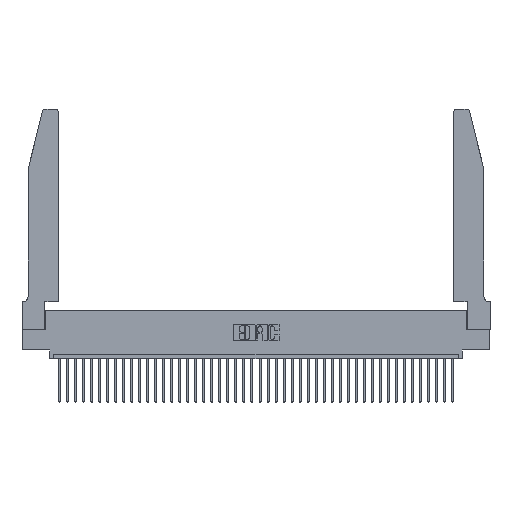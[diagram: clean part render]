
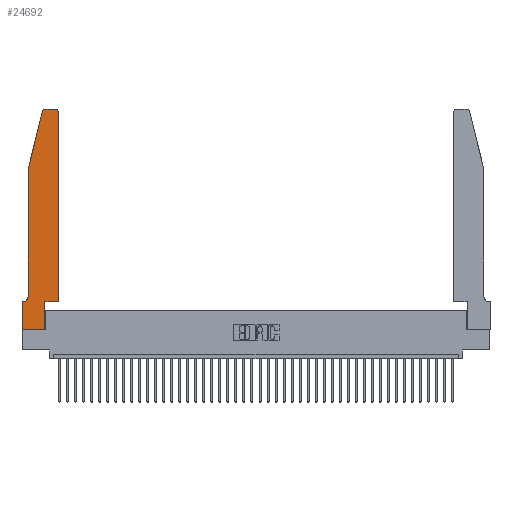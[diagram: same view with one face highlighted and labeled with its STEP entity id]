
A CAD part, top view. The second image highlights one B-rep face of the part: STEP entity #24692.
In plain terms, the highlighted planar face has unit normal (0, 0, 1).
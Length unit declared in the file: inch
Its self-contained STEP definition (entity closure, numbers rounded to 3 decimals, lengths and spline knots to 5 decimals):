
#1592 = VERTEX_POINT ( 'NONE', #25373 ) ;
#1795 = DIRECTION ( 'NONE',  ( 1., 0., 0. ) ) ;
#1961 = VERTEX_POINT ( 'NONE', #6447 ) ;
#2151 = CARTESIAN_POINT ( 'NONE',  ( 0.4205, 2.72, 0.37 ) ) ;
#2471 = CARTESIAN_POINT ( 'NONE',  ( 0.0755, 0.42, 0.37 ) ) ;
#2790 = LINE ( 'NONE', #35418, #9738 ) ;
#3398 = LINE ( 'NONE', #11113, #10912 ) ;
#3417 = ORIENTED_EDGE ( 'NONE', *, *, #31023, .T. ) ;
#3497 = VECTOR ( 'NONE', #39187, 39.37008 ) ;
#4073 = AXIS2_PLACEMENT_3D ( 'NONE', #36904, #4329, #7542 ) ;
#4329 = DIRECTION ( 'NONE',  ( 0., 0., 1. ) ) ;
#6447 = CARTESIAN_POINT ( 'NONE',  ( 0.0055, 0.35, 0.37 ) ) ;
#7184 = EDGE_CURVE ( 'NONE', #39965, #19080, #30500, .T. ) ;
#7542 = DIRECTION ( 'NONE',  ( 1., 0., 0. ) ) ;
#8262 = DIRECTION ( 'NONE',  ( 0., 0., 1. ) ) ;
#8301 = LINE ( 'NONE', #34296, #31265 ) ;
#8438 = DIRECTION ( 'NONE',  ( 1., 0., 0. ) ) ;
#8507 = DIRECTION ( 'NONE',  ( 0., -1., 0. ) ) ;
#8830 = CIRCLE ( 'NONE', #4073, 0.03 ) ;
#9182 = ORIENTED_EDGE ( 'NONE', *, *, #26389, .T. ) ;
#9738 = VECTOR ( 'NONE', #22558, 39.37008 ) ;
#9892 = CARTESIAN_POINT ( 'NONE',  ( 0.0755, 2., 0.37 ) ) ;
#10558 = VERTEX_POINT ( 'NONE', #12761 ) ;
#10912 = VECTOR ( 'NONE', #26677, 39.37008 ) ;
#10990 = LINE ( 'NONE', #30282, #27464 ) ;
#11113 = CARTESIAN_POINT ( 'NONE',  ( 0.4505, 0.35, 0.37 ) ) ;
#11915 = CARTESIAN_POINT ( 'NONE',  ( 0.284, 2.75, 0.37 ) ) ;
#12387 = ORIENTED_EDGE ( 'NONE', *, *, #39981, .T. ) ;
#12761 = CARTESIAN_POINT ( 'NONE',  ( 0.4505, 2.72, 0.37 ) ) ;
#13233 = CARTESIAN_POINT ( 'NONE',  ( 0., 0., 0.37 ) ) ;
#13507 = VECTOR ( 'NONE', #8507, 39.37008 ) ;
#13858 = AXIS2_PLACEMENT_3D ( 'NONE', #2151, #27553, #8438 ) ;
#14632 = AXIS2_PLACEMENT_3D ( 'NONE', #34479, #18452, #25092 ) ;
#15091 = CARTESIAN_POINT ( 'NONE',  ( 0., 0.35, 0.37 ) ) ;
#15648 = ORIENTED_EDGE ( 'NONE', *, *, #28851, .T. ) ;
#16518 = CARTESIAN_POINT ( 'NONE',  ( 0.25487, 2.72718, 0.37 ) ) ;
#17806 = EDGE_CURVE ( 'NONE', #23281, #10558, #3398, .T. ) ;
#17874 = LINE ( 'NONE', #36622, #32758 ) ;
#18004 = CARTESIAN_POINT ( 'NONE',  ( 0., 0., 0.37 ) ) ;
#18163 = CARTESIAN_POINT ( 'NONE',  ( 0.4505, 0.35, 0.37 ) ) ;
#18452 = DIRECTION ( 'NONE',  ( 0., 0., -1. ) ) ;
#18645 = ORIENTED_EDGE ( 'NONE', *, *, #27045, .T. ) ;
#18947 = CIRCLE ( 'NONE', #14632, 0.07 ) ;
#19080 = VERTEX_POINT ( 'NONE', #2471 ) ;
#19189 = EDGE_CURVE ( 'NONE', #30478, #39965, #17874, .T. ) ;
#19317 = CARTESIAN_POINT ( 'NONE',  ( 0.2865, 0.35, 0.37 ) ) ;
#19627 = LINE ( 'NONE', #39308, #32118 ) ;
#19789 = AXIS2_PLACEMENT_3D ( 'NONE', #15091, #8262, #1795 ) ;
#20013 = LINE ( 'NONE', #13233, #3497 ) ;
#20173 = CIRCLE ( 'NONE', #13858, 0.03 ) ;
#20336 = ORIENTED_EDGE ( 'NONE', *, *, #17806, .T. ) ;
#20434 = VERTEX_POINT ( 'NONE', #40212 ) ;
#20573 = VERTEX_POINT ( 'NONE', #18004 ) ;
#20961 = DIRECTION ( 'NONE',  ( 1., 0., 0. ) ) ;
#21600 = EDGE_CURVE ( 'NONE', #1592, #28769, #19627, .T. ) ;
#22558 = DIRECTION ( 'NONE',  ( -1., 0., 0. ) ) ;
#23281 = VERTEX_POINT ( 'NONE', #18163 ) ;
#23742 = DIRECTION ( 'NONE',  ( -0.239, -0.971, 0. ) ) ;
#24692 = ADVANCED_FACE ( 'NONE', ( #34099 ), #40645, .T. ) ;
#25053 = DIRECTION ( 'NONE',  ( 1., 0., 0. ) ) ;
#25092 = DIRECTION ( 'NONE',  ( -1., 0., 0. ) ) ;
#25373 = CARTESIAN_POINT ( 'NONE',  ( 0.2865, 0., 0.37 ) ) ;
#25801 = VERTEX_POINT ( 'NONE', #26872 ) ;
#26389 = EDGE_CURVE ( 'NONE', #20434, #20573, #20013, .T. ) ;
#26576 = DIRECTION ( 'NONE',  ( 0., 1., 0. ) ) ;
#26677 = DIRECTION ( 'NONE',  ( 0., 1., 0. ) ) ;
#26872 = CARTESIAN_POINT ( 'NONE',  ( 0.4205, 2.75, 0.37 ) ) ;
#27045 = EDGE_CURVE ( 'NONE', #28769, #23281, #10990, .T. ) ;
#27464 = VECTOR ( 'NONE', #20961, 39.37008 ) ;
#27553 = DIRECTION ( 'NONE',  ( 0., 0., 1. ) ) ;
#27750 = VECTOR ( 'NONE', #38518, 39.37008 ) ;
#27829 = EDGE_CURVE ( 'NONE', #19080, #1961, #18947, .T. ) ;
#27870 = ORIENTED_EDGE ( 'NONE', *, *, #27829, .T. ) ;
#28499 = ORIENTED_EDGE ( 'NONE', *, *, #7184, .T. ) ;
#28769 = VERTEX_POINT ( 'NONE', #19317 ) ;
#28851 = EDGE_CURVE ( 'NONE', #35523, #30478, #8830, .T. ) ;
#29299 = EDGE_CURVE ( 'NONE', #25801, #35523, #2790, .T. ) ;
#30282 = CARTESIAN_POINT ( 'NONE',  ( 0.4505, 0.35, 0.37 ) ) ;
#30478 = VERTEX_POINT ( 'NONE', #16518 ) ;
#30500 = LINE ( 'NONE', #40474, #13507 ) ;
#31023 = EDGE_CURVE ( 'NONE', #20573, #1592, #8301, .T. ) ;
#31265 = VECTOR ( 'NONE', #25053, 39.37008 ) ;
#31671 = EDGE_CURVE ( 'NONE', #10558, #25801, #20173, .T. ) ;
#31714 = ORIENTED_EDGE ( 'NONE', *, *, #21600, .T. ) ;
#32118 = VECTOR ( 'NONE', #26576, 39.37008 ) ;
#32629 = ORIENTED_EDGE ( 'NONE', *, *, #19189, .T. ) ;
#32758 = VECTOR ( 'NONE', #23742, 39.37008 ) ;
#34099 = FACE_OUTER_BOUND ( 'NONE', #38593, .T. ) ;
#34296 = CARTESIAN_POINT ( 'NONE',  ( 0., 0., 0.37 ) ) ;
#34346 = ORIENTED_EDGE ( 'NONE', *, *, #31671, .T. ) ;
#34479 = CARTESIAN_POINT ( 'NONE',  ( 0.0055, 0.42, 0.37 ) ) ;
#35418 = CARTESIAN_POINT ( 'NONE',  ( 0.2605, 2.75, 0.37 ) ) ;
#35523 = VERTEX_POINT ( 'NONE', #11915 ) ;
#36561 = ORIENTED_EDGE ( 'NONE', *, *, #29299, .T. ) ;
#36622 = CARTESIAN_POINT ( 'NONE',  ( 0.0755, 2., 0.37 ) ) ;
#36904 = CARTESIAN_POINT ( 'NONE',  ( 0.284, 2.72, 0.37 ) ) ;
#37779 = LINE ( 'NONE', #38658, #27750 ) ;
#38518 = DIRECTION ( 'NONE',  ( -1., 0., 0. ) ) ;
#38593 = EDGE_LOOP ( 'NONE', ( #36561, #15648, #32629, #28499, #27870, #12387, #9182, #3417, #31714, #18645, #20336, #34346 ) ) ;
#38658 = CARTESIAN_POINT ( 'NONE',  ( 0.0755, 0.35, 0.37 ) ) ;
#39187 = DIRECTION ( 'NONE',  ( 0., -1., 0. ) ) ;
#39308 = CARTESIAN_POINT ( 'NONE',  ( 0.2865, 0.35, 0.37 ) ) ;
#39965 = VERTEX_POINT ( 'NONE', #9892 ) ;
#39981 = EDGE_CURVE ( 'NONE', #1961, #20434, #37779, .T. ) ;
#40212 = CARTESIAN_POINT ( 'NONE',  ( 0., 0.35, 0.37 ) ) ;
#40474 = CARTESIAN_POINT ( 'NONE',  ( 0.0755, 2., 0.37 ) ) ;
#40645 = PLANE ( 'NONE',  #19789 ) ;
